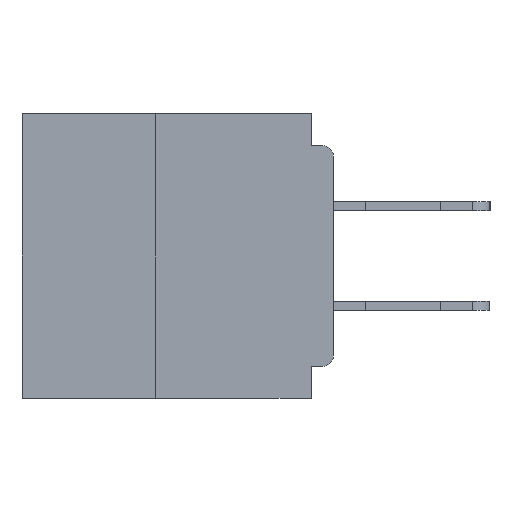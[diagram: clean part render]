
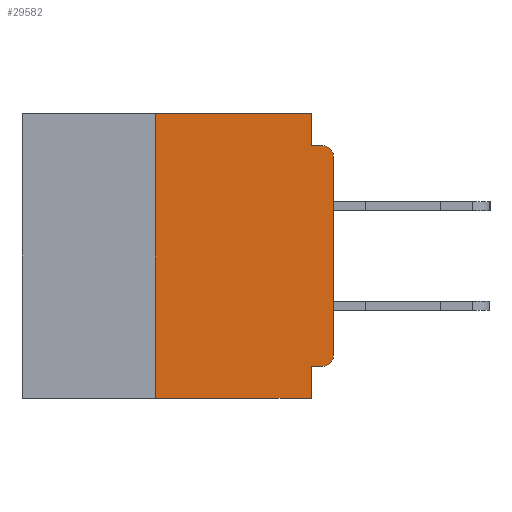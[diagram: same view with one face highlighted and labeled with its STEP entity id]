
A CAD part, left-side view. The second image highlights one B-rep face of the part: STEP entity #29582.
In plain terms, the highlighted planar face has unit normal (-1, 0, 0).
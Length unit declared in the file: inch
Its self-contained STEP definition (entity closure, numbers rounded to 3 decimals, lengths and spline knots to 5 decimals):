
#128 = CARTESIAN_POINT ( 'NONE',  ( 0., 0.031, -0.4 ) ) ;
#697 = VERTEX_POINT ( 'NONE', #38522 ) ;
#1039 = CARTESIAN_POINT ( 'NONE',  ( 0., 0.015, -0.06 ) ) ;
#2174 = VERTEX_POINT ( 'NONE', #22422 ) ;
#2518 = ORIENTED_EDGE ( 'NONE', *, *, #45201, .F. ) ;
#2746 = FACE_OUTER_BOUND ( 'NONE', #4103, .T. ) ;
#2763 = LINE ( 'NONE', #6277, #30056 ) ;
#3371 = EDGE_CURVE ( 'NONE', #42944, #4405, #46958, .T. ) ;
#3443 = VERTEX_POINT ( 'NONE', #40767 ) ;
#4044 = VERTEX_POINT ( 'NONE', #33439 ) ;
#4103 = EDGE_LOOP ( 'NONE', ( #40304, #14233, #45382, #2518, #39348, #47484, #18086, #45482, #8871, #11572 ) ) ;
#4232 = LINE ( 'NONE', #21980, #41075 ) ;
#4405 = VERTEX_POINT ( 'NONE', #31682 ) ;
#4784 = DIRECTION ( 'NONE',  ( 0., 0., -1. ) ) ;
#4828 = VECTOR ( 'NONE', #36270, 39.37008 ) ;
#5100 = VERTEX_POINT ( 'NONE', #31720 ) ;
#6277 = CARTESIAN_POINT ( 'NONE',  ( 0., 0.031, 0. ) ) ;
#6624 = CARTESIAN_POINT ( 'NONE',  ( 0., 0., -0.355 ) ) ;
#7523 = CARTESIAN_POINT ( 'NONE',  ( 0., 0.015, -0.34 ) ) ;
#8241 = AXIS2_PLACEMENT_3D ( 'NONE', #7523, #33340, #11243 ) ;
#8871 = ORIENTED_EDGE ( 'NONE', *, *, #47370, .F. ) ;
#9409 = LINE ( 'NONE', #21705, #19315 ) ;
#9816 = VERTEX_POINT ( 'NONE', #10769 ) ;
#10769 = CARTESIAN_POINT ( 'NONE',  ( 0., 0.031, -0.045 ) ) ;
#11243 = DIRECTION ( 'NONE',  ( 0., 0., -1. ) ) ;
#11572 = ORIENTED_EDGE ( 'NONE', *, *, #3371, .T. ) ;
#11609 = CARTESIAN_POINT ( 'NONE',  ( 0., 0.437, 0. ) ) ;
#12296 = CARTESIAN_POINT ( 'NONE',  ( 0., 0.25, -0.4 ) ) ;
#12584 = VECTOR ( 'NONE', #23312, 39.37008 ) ;
#12813 = DIRECTION ( 'NONE',  ( 0., 0., 1. ) ) ;
#14233 = ORIENTED_EDGE ( 'NONE', *, *, #23357, .T. ) ;
#14387 = CARTESIAN_POINT ( 'NONE',  ( 0., 0.015, -0.355 ) ) ;
#14690 = LINE ( 'NONE', #6624, #4828 ) ;
#16227 = DIRECTION ( 'NONE',  ( 0., -1., 0. ) ) ;
#18086 = ORIENTED_EDGE ( 'NONE', *, *, #33049, .T. ) ;
#18951 = PLANE ( 'NONE',  #35047 ) ;
#19103 = DIRECTION ( 'NONE',  ( 0., 0., -1. ) ) ;
#19315 = VECTOR ( 'NONE', #39853, 39.37008 ) ;
#19318 = VECTOR ( 'NONE', #12813, 39.37008 ) ;
#20902 = VERTEX_POINT ( 'NONE', #128 ) ;
#21705 = CARTESIAN_POINT ( 'NONE',  ( 0., 0.437, 0. ) ) ;
#21980 = CARTESIAN_POINT ( 'NONE',  ( 0., 0.437, -0.4 ) ) ;
#22422 = CARTESIAN_POINT ( 'NONE',  ( 0., 0.015, -0.045 ) ) ;
#23312 = DIRECTION ( 'NONE',  ( 0., 0., 1. ) ) ;
#23357 = EDGE_CURVE ( 'NONE', #3443, #2174, #28405, .T. ) ;
#23993 = EDGE_CURVE ( 'NONE', #4405, #3443, #39574, .T. ) ;
#25720 = EDGE_CURVE ( 'NONE', #4044, #20902, #37150, .T. ) ;
#27058 = DIRECTION ( 'NONE',  ( -1., 0., 0. ) ) ;
#27260 = CARTESIAN_POINT ( 'NONE',  ( 0., 0., -0.045 ) ) ;
#28405 = CIRCLE ( 'NONE', #29075, 0.015 ) ;
#28650 = VECTOR ( 'NONE', #34290, 39.37008 ) ;
#29075 = AXIS2_PLACEMENT_3D ( 'NONE', #1039, #27058, #4784 ) ;
#29116 = VECTOR ( 'NONE', #16227, 39.37008 ) ;
#29127 = LINE ( 'NONE', #41977, #19318 ) ;
#29582 = ADVANCED_FACE ( 'NONE', ( #2746 ), #18951, .F. ) ;
#30056 = VECTOR ( 'NONE', #46569, 39.37008 ) ;
#31027 = VERTEX_POINT ( 'NONE', #12296 ) ;
#31682 = CARTESIAN_POINT ( 'NONE',  ( 0., 0., -0.34 ) ) ;
#31720 = CARTESIAN_POINT ( 'NONE',  ( 0., 0.25, 0. ) ) ;
#33005 = DIRECTION ( 'NONE',  ( 0., -1., 0. ) ) ;
#33049 = EDGE_CURVE ( 'NONE', #31027, #20902, #4232, .T. ) ;
#33340 = DIRECTION ( 'NONE',  ( -1., 0., 0. ) ) ;
#33439 = CARTESIAN_POINT ( 'NONE',  ( 0., 0.031, -0.355 ) ) ;
#34290 = DIRECTION ( 'NONE',  ( 0., 0., -1. ) ) ;
#34669 = EDGE_CURVE ( 'NONE', #9816, #2174, #38750, .T. ) ;
#35047 = AXIS2_PLACEMENT_3D ( 'NONE', #11609, #40974, #19103 ) ;
#36270 = DIRECTION ( 'NONE',  ( 0., 1., 0. ) ) ;
#37150 = LINE ( 'NONE', #45214, #28650 ) ;
#37944 = EDGE_CURVE ( 'NONE', #31027, #5100, #29127, .T. ) ;
#38522 = CARTESIAN_POINT ( 'NONE',  ( 0., 0.031, 0. ) ) ;
#38750 = LINE ( 'NONE', #27260, #29116 ) ;
#39348 = ORIENTED_EDGE ( 'NONE', *, *, #42411, .F. ) ;
#39574 = LINE ( 'NONE', #45061, #12584 ) ;
#39853 = DIRECTION ( 'NONE',  ( 0., -1., 0. ) ) ;
#40304 = ORIENTED_EDGE ( 'NONE', *, *, #23993, .T. ) ;
#40767 = CARTESIAN_POINT ( 'NONE',  ( 0., 0., -0.06 ) ) ;
#40974 = DIRECTION ( 'NONE',  ( 1., 0., 0. ) ) ;
#41075 = VECTOR ( 'NONE', #33005, 39.37008 ) ;
#41977 = CARTESIAN_POINT ( 'NONE',  ( 0., 0.25, -0.4 ) ) ;
#42411 = EDGE_CURVE ( 'NONE', #5100, #697, #9409, .T. ) ;
#42944 = VERTEX_POINT ( 'NONE', #14387 ) ;
#45061 = CARTESIAN_POINT ( 'NONE',  ( 0., 0., 0. ) ) ;
#45201 = EDGE_CURVE ( 'NONE', #697, #9816, #2763, .T. ) ;
#45214 = CARTESIAN_POINT ( 'NONE',  ( 0., 0.031, -0.4 ) ) ;
#45382 = ORIENTED_EDGE ( 'NONE', *, *, #34669, .F. ) ;
#45482 = ORIENTED_EDGE ( 'NONE', *, *, #25720, .F. ) ;
#46569 = DIRECTION ( 'NONE',  ( 0., 0., -1. ) ) ;
#46958 = CIRCLE ( 'NONE', #8241, 0.015 ) ;
#47370 = EDGE_CURVE ( 'NONE', #42944, #4044, #14690, .T. ) ;
#47484 = ORIENTED_EDGE ( 'NONE', *, *, #37944, .F. ) ;
